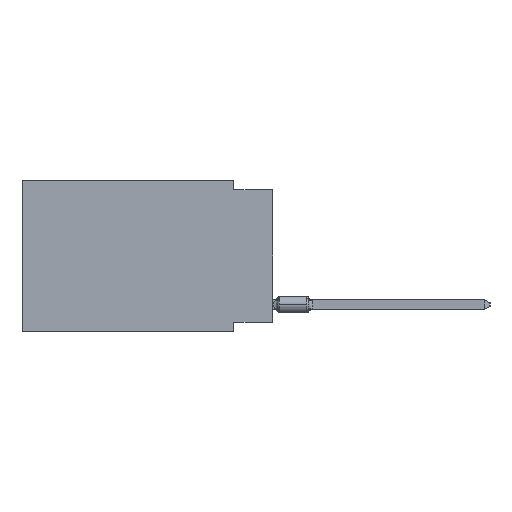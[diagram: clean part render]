
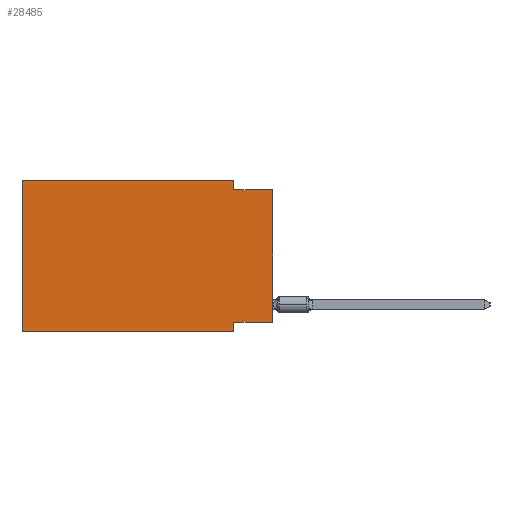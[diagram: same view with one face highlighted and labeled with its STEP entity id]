
A CAD part, left-side view. The second image highlights one B-rep face of the part: STEP entity #28485.
In plain terms, the highlighted planar face has unit normal (-1, 0, 0).
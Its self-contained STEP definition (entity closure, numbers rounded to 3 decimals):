
#121 = CARTESIAN_POINT ( 'NONE',  ( 0., 0., -0.635 ) ) ;
#980 = DIRECTION ( 'NONE',  ( 0., 0., -1. ) ) ;
#1255 = CARTESIAN_POINT ( 'NONE',  ( 0., 2.54, -9.906 ) ) ;
#1344 = VERTEX_POINT ( 'NONE', #42921 ) ;
#1546 = LINE ( 'NONE', #1255, #39769 ) ;
#1851 = DIRECTION ( 'NONE',  ( 0., 1., 0. ) ) ;
#2571 = LINE ( 'NONE', #40663, #21197 ) ;
#3161 = VECTOR ( 'NONE', #6366, 1000. ) ;
#3466 = DIRECTION ( 'NONE',  ( 0., 0., -1. ) ) ;
#3869 = DIRECTION ( 'NONE',  ( 0., -1., 0. ) ) ;
#4568 = EDGE_LOOP ( 'NONE', ( #33118, #19917, #50284, #18639, #52501, #44203, #7401, #55043 ) ) ;
#6366 = DIRECTION ( 'NONE',  ( 0., -1., 0. ) ) ;
#6405 = EDGE_CURVE ( 'NONE', #34397, #24764, #2571, .T. ) ;
#7401 = ORIENTED_EDGE ( 'NONE', *, *, #44013, .F. ) ;
#7475 = CARTESIAN_POINT ( 'NONE',  ( 0., 0., -0.635 ) ) ;
#10156 = CARTESIAN_POINT ( 'NONE',  ( 0., 2.54, -0.635 ) ) ;
#11149 = DIRECTION ( 'NONE',  ( 0., 0., -1. ) ) ;
#11344 = EDGE_CURVE ( 'NONE', #1344, #54917, #47208, .T. ) ;
#13339 = VECTOR ( 'NONE', #30164, 1000. ) ;
#14579 = VECTOR ( 'NONE', #38577, 1000. ) ;
#15495 = FACE_OUTER_BOUND ( 'NONE', #4568, .T. ) ;
#15858 = VERTEX_POINT ( 'NONE', #53477 ) ;
#16328 = DIRECTION ( 'NONE',  ( 1., 0., 0. ) ) ;
#16882 = VECTOR ( 'NONE', #48378, 1000. ) ;
#17953 = CARTESIAN_POINT ( 'NONE',  ( 0., 16.383, 0. ) ) ;
#18314 = CARTESIAN_POINT ( 'NONE',  ( 0., 16.383, 0. ) ) ;
#18639 = ORIENTED_EDGE ( 'NONE', *, *, #48192, .F. ) ;
#19503 = CARTESIAN_POINT ( 'NONE',  ( 0., 16.383, -9.906 ) ) ;
#19917 = ORIENTED_EDGE ( 'NONE', *, *, #45163, .F. ) ;
#20643 = CARTESIAN_POINT ( 'NONE',  ( 0., 16.383, -9.906 ) ) ;
#21137 = CARTESIAN_POINT ( 'NONE',  ( 0., 0., 0. ) ) ;
#21197 = VECTOR ( 'NONE', #11149, 1000. ) ;
#21473 = VERTEX_POINT ( 'NONE', #20643 ) ;
#23034 = CARTESIAN_POINT ( 'NONE',  ( 0., 0., -9.271 ) ) ;
#23807 = AXIS2_PLACEMENT_3D ( 'NONE', #24623, #16328, #3466 ) ;
#24623 = CARTESIAN_POINT ( 'NONE',  ( 0., 16.383, 0. ) ) ;
#24764 = VERTEX_POINT ( 'NONE', #10156 ) ;
#26491 = VERTEX_POINT ( 'NONE', #17953 ) ;
#28485 = ADVANCED_FACE ( 'NONE', ( #15495 ), #54995, .F. ) ;
#30164 = DIRECTION ( 'NONE',  ( 0., -1., 0. ) ) ;
#33118 = ORIENTED_EDGE ( 'NONE', *, *, #11344, .T. ) ;
#33456 = EDGE_CURVE ( 'NONE', #21473, #15858, #53604, .T. ) ;
#34397 = VERTEX_POINT ( 'NONE', #46188 ) ;
#35095 = VECTOR ( 'NONE', #3869, 1000. ) ;
#35122 = EDGE_CURVE ( 'NONE', #1344, #54918, #45083, .T. ) ;
#35829 = LINE ( 'NONE', #45008, #35095 ) ;
#38577 = DIRECTION ( 'NONE',  ( 0., 0., 1. ) ) ;
#39769 = VECTOR ( 'NONE', #980, 1000. ) ;
#40663 = CARTESIAN_POINT ( 'NONE',  ( 0., 2.54, 0. ) ) ;
#42921 = CARTESIAN_POINT ( 'NONE',  ( 0., 0., -9.271 ) ) ;
#44013 = EDGE_CURVE ( 'NONE', #54918, #15858, #1546, .T. ) ;
#44203 = ORIENTED_EDGE ( 'NONE', *, *, #33456, .T. ) ;
#45008 = CARTESIAN_POINT ( 'NONE',  ( 0., 16.383, 0. ) ) ;
#45083 = LINE ( 'NONE', #23034, #46633 ) ;
#45163 = EDGE_CURVE ( 'NONE', #24764, #54917, #52511, .T. ) ;
#46188 = CARTESIAN_POINT ( 'NONE',  ( 0., 2.54, 0. ) ) ;
#46633 = VECTOR ( 'NONE', #1851, 1000. ) ;
#47208 = LINE ( 'NONE', #21137, #14579 ) ;
#47534 = CARTESIAN_POINT ( 'NONE',  ( 0., 2.54, -9.271 ) ) ;
#48192 = EDGE_CURVE ( 'NONE', #26491, #34397, #35829, .T. ) ;
#48378 = DIRECTION ( 'NONE',  ( 0., 0., 1. ) ) ;
#48573 = EDGE_CURVE ( 'NONE', #21473, #26491, #48953, .T. ) ;
#48953 = LINE ( 'NONE', #18314, #16882 ) ;
#50284 = ORIENTED_EDGE ( 'NONE', *, *, #6405, .F. ) ;
#52501 = ORIENTED_EDGE ( 'NONE', *, *, #48573, .F. ) ;
#52511 = LINE ( 'NONE', #121, #13339 ) ;
#53477 = CARTESIAN_POINT ( 'NONE',  ( 0., 2.54, -9.906 ) ) ;
#53604 = LINE ( 'NONE', #19503, #3161 ) ;
#54917 = VERTEX_POINT ( 'NONE', #7475 ) ;
#54918 = VERTEX_POINT ( 'NONE', #47534 ) ;
#54995 = PLANE ( 'NONE',  #23807 ) ;
#55043 = ORIENTED_EDGE ( 'NONE', *, *, #35122, .F. ) ;
